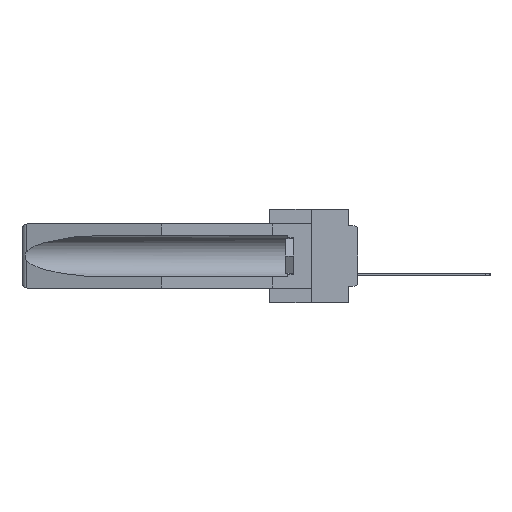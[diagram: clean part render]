
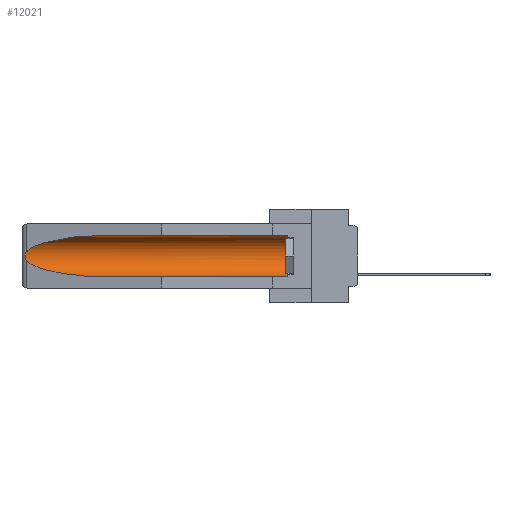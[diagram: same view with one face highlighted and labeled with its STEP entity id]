
A CAD part, left-side view. The second image highlights one B-rep face of the part: STEP entity #12021.
In plain terms, the highlighted cylindrical face has radius 2.857 mm (diameter 5.715 mm), a partial arc.
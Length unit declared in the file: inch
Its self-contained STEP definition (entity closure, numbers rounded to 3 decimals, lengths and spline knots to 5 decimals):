
#30 = ORIENTED_EDGE ( 'NONE', *, *, #21940, .T. ) ;
#385 = VERTEX_POINT ( 'NONE', #4979 ) ;
#1064 = DIRECTION ( 'NONE',  ( 0., 0., 1. ) ) ;
#1535 = CARTESIAN_POINT ( 'NONE',  ( 0.26537, 1.52718, -0.14972 ) ) ;
#1578 = CARTESIAN_POINT ( 'NONE',  ( 0.25451, 1.48313, -0.09465 ) ) ;
#3203 =( BOUNDED_CURVE ( )  B_SPLINE_CURVE ( 3, ( #15360, #18110, #1578, #20810 ),
 .UNSPECIFIED., .F., .F. ) 
 B_SPLINE_CURVE_WITH_KNOTS ( ( 4, 4 ),
 ( 4.71239, 6.08839 ),
 .UNSPECIFIED. ) 
 CURVE ( )  GEOMETRIC_REPRESENTATION_ITEM ( )  RATIONAL_B_SPLINE_CURVE ( ( 1., 0.848, 0.848, 1. ) ) 
 REPRESENTATION_ITEM ( '' )  );
#3395 = AXIS2_PLACEMENT_3D ( 'NONE', #24803, #16688, #5714 ) ;
#4075 = CYLINDRICAL_SURFACE ( 'NONE', #3395, 0.1125 ) ;
#4312 = CARTESIAN_POINT ( 'NONE',  ( 0.2673, 1.5327, -0.16383 ) ) ;
#4581 = ORIENTED_EDGE ( 'NONE', *, *, #8787, .T. ) ;
#4979 = CARTESIAN_POINT ( 'NONE',  ( 0.155, 0.126, -0.284 ) ) ;
#5714 = DIRECTION ( 'NONE',  ( 0., 0., 1. ) ) ;
#6345 = CARTESIAN_POINT ( 'NONE',  ( 0.155, 0.126, -0.059 ) ) ;
#7131 = CARTESIAN_POINT ( 'NONE',  ( 0.2675, 1.53308, -0.17534 ) ) ;
#7183 = CARTESIAN_POINT ( 'NONE',  ( 0.21114, 1.30732, -0.284 ) ) ;
#7678 = EDGE_CURVE ( 'NONE', #24897, #31630, #28208, .T. ) ;
#8066 = DIRECTION ( 'NONE',  ( 0., 1., 0. ) ) ;
#8787 = EDGE_CURVE ( 'NONE', #31630, #14608, #34767, .T. ) ;
#9090 = DIRECTION ( 'NONE',  ( 0., 1., 0. ) ) ;
#9305 = CARTESIAN_POINT ( 'NONE',  ( 0.155, 1.07973, -0.059 ) ) ;
#9929 = CARTESIAN_POINT ( 'NONE',  ( 0.26655, 1.53094, -0.18657 ) ) ;
#11263 = AXIS2_PLACEMENT_3D ( 'NONE', #33695, #17609, #1064 ) ;
#11800 = VECTOR ( 'NONE', #8066, 39.37008 ) ;
#11823 = CARTESIAN_POINT ( 'NONE',  ( 0.155, -0.30754, -0.059 ) ) ;
#12021 = ADVANCED_FACE ( 'NONE', ( #25874 ), #4075, .F. ) ;
#12355 = EDGE_CURVE ( 'NONE', #32313, #24897, #3203, .T. ) ;
#12477 = ORIENTED_EDGE ( 'NONE', *, *, #12780, .T. ) ;
#12641 = CARTESIAN_POINT ( 'NONE',  ( 0.26537, 1.52718, -0.19328 ) ) ;
#12780 = EDGE_CURVE ( 'NONE', #385, #30724, #32214, .T. ) ;
#14608 = VERTEX_POINT ( 'NONE', #22343 ) ;
#14769 = ORIENTED_EDGE ( 'NONE', *, *, #7678, .T. ) ;
#15360 = CARTESIAN_POINT ( 'NONE',  ( 0.155, 1.07973, -0.059 ) ) ;
#16632 = CARTESIAN_POINT ( 'NONE',  ( 0.26537, 1.52718, -0.14972 ) ) ;
#16688 = DIRECTION ( 'NONE',  ( 0., 1., 0. ) ) ;
#17609 = DIRECTION ( 'NONE',  ( 0., -1., 0. ) ) ;
#18110 = CARTESIAN_POINT ( 'NONE',  ( 0.21114, 1.30732, -0.059 ) ) ;
#18113 = CARTESIAN_POINT ( 'NONE',  ( 0.25451, 1.48313, -0.24835 ) ) ;
#20761 = CARTESIAN_POINT ( 'NONE',  ( 0.26654, 1.53092, -0.15636 ) ) ;
#20810 = CARTESIAN_POINT ( 'NONE',  ( 0.26537, 1.52718, -0.14972 ) ) ;
#21916 = ORIENTED_EDGE ( 'NONE', *, *, #22747, .F. ) ;
#21940 = EDGE_CURVE ( 'NONE', #30724, #32313, #30104, .T. ) ;
#22343 = CARTESIAN_POINT ( 'NONE',  ( 0.155, 1.07973, -0.284 ) ) ;
#22747 = EDGE_CURVE ( 'NONE', #385, #14608, #26245, .T. ) ;
#22966 = VECTOR ( 'NONE', #9090, 39.37008 ) ;
#23476 = CARTESIAN_POINT ( 'NONE',  ( 0.2675, 1.53308, -0.16763 ) ) ;
#24803 = CARTESIAN_POINT ( 'NONE',  ( 0.155, -0.30754, -0.1715 ) ) ;
#24897 = VERTEX_POINT ( 'NONE', #16632 ) ;
#25372 = EDGE_LOOP ( 'NONE', ( #25380, #14769, #4581, #21916, #12477, #30 ) ) ;
#25380 = ORIENTED_EDGE ( 'NONE', *, *, #12355, .T. ) ;
#25874 = FACE_OUTER_BOUND ( 'NONE', #25372, .T. ) ;
#26157 = CARTESIAN_POINT ( 'NONE',  ( 0.2673, 1.53269, -0.17917 ) ) ;
#26210 = CARTESIAN_POINT ( 'NONE',  ( 0.155, 1.07973, -0.284 ) ) ;
#26245 = LINE ( 'NONE', #35014, #11800 ) ;
#28208 = B_SPLINE_CURVE_WITH_KNOTS ( 'NONE', 3,
 ( #1535, #31469, #20761, #4312, #23476, #7131, #26157, #9929, #28895, #12641 ),
 .UNSPECIFIED., .F., .F.,
 ( 4, 2, 2, 2, 4 ),
 ( 0., 0.00029, 0.00058, 0.00087, 0.00117 ),
 .UNSPECIFIED. ) ;
#28895 = CARTESIAN_POINT ( 'NONE',  ( 0.26597, 1.5296, -0.19026 ) ) ;
#30104 = LINE ( 'NONE', #11823, #22966 ) ;
#30724 = VERTEX_POINT ( 'NONE', #6345 ) ;
#31469 = CARTESIAN_POINT ( 'NONE',  ( 0.26597, 1.52961, -0.15275 ) ) ;
#31630 = VERTEX_POINT ( 'NONE', #33604 ) ;
#32214 = CIRCLE ( 'NONE', #11263, 0.1125 ) ;
#32313 = VERTEX_POINT ( 'NONE', #9305 ) ;
#33604 = CARTESIAN_POINT ( 'NONE',  ( 0.26537, 1.52718, -0.19328 ) ) ;
#33695 = CARTESIAN_POINT ( 'NONE',  ( 0.155, 0.126, -0.1715 ) ) ;
#34191 = CARTESIAN_POINT ( 'NONE',  ( 0.26537, 1.52718, -0.19328 ) ) ;
#34767 =( BOUNDED_CURVE ( )  B_SPLINE_CURVE ( 3, ( #34191, #18113, #7183, #26210 ),
 .UNSPECIFIED., .F., .F. ) 
 B_SPLINE_CURVE_WITH_KNOTS ( ( 4, 4 ),
 ( 0.1948, 1.5708 ),
 .UNSPECIFIED. ) 
 CURVE ( )  GEOMETRIC_REPRESENTATION_ITEM ( )  RATIONAL_B_SPLINE_CURVE ( ( 1., 0.848, 0.848, 1. ) ) 
 REPRESENTATION_ITEM ( '' )  );
#35014 = CARTESIAN_POINT ( 'NONE',  ( 0.155, -0.30754, -0.284 ) ) ;
